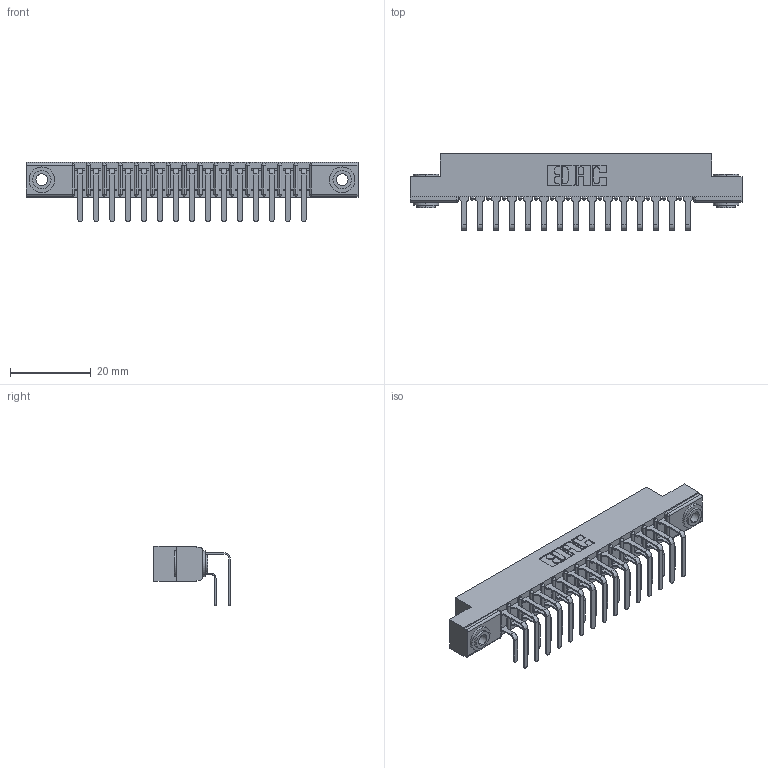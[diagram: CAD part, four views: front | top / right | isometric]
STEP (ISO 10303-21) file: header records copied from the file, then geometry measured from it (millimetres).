
FILE_DESCRIPTION (( 'STEP AP203' ), '1' );
FILE_NAME ('307-030-458-203.STEP', '2020-09-29T10:01:16', ( '' ), ( '' ), 'SwSTEP 2.0', 'SolidWorks 2020', '' );
FILE_SCHEMA (( 'CONFIG_CONTROL_DESIGN' ));
Length unit declared in the file: inch
Products named in the file (5): 307 Part_.156 Dia Mounting Holes; 307-030-458-203; 307-290-001_558 559 - 1 (Single); 345-250-002_345-250-002-102; 307-290-001_558 - 2 (Single)
Assembly tree (33 placements, depth 2):
  307-030-458-203
    307 Part_.156 Dia Mounting Holes
    307-290-001_558 559 - 1 (Single)  x15
    307-290-001_558 - 2 (Single)  x15
    345-250-002_345-250-002-102  x2
Bounding box: 82.45 x 18.96 x 14.81 mm (x, y, z)
Volume: 5528.1 mm3; surface area: 10394.9 mm2
Topology: 33 solids, 33 shells, 1686 faces, 4695 edges, 3042 vertices
Faces by surface type: plane 1084, cylinder 562, sphere 32, cone 8
Entity records: 19180 total; most frequent: CARTESIAN_POINT 3130, DIRECTION 3091, ORIENTED_EDGE 3090, EDGE_CURVE 1545, LINE 1165, VECTOR 1165, VERTEX_POINT 1002, AXIS2_PLACEMENT_3D 963
